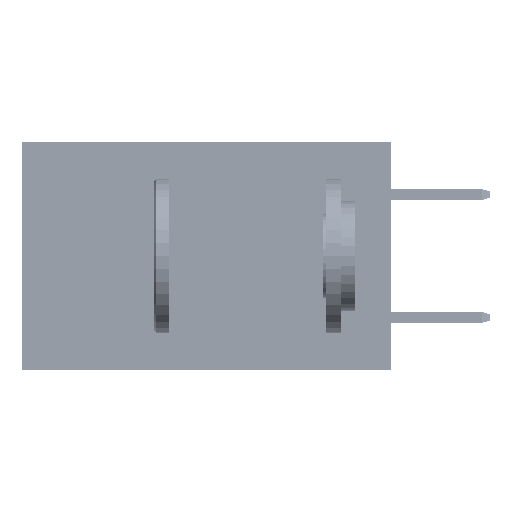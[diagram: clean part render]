
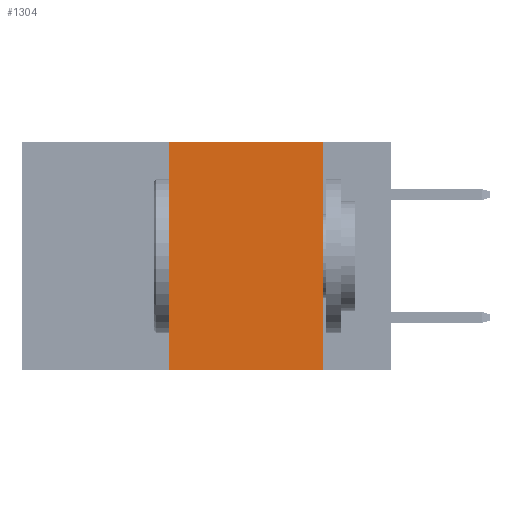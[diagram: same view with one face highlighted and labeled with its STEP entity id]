
A CAD part, left-side view. The second image highlights one B-rep face of the part: STEP entity #1304.
In plain terms, the highlighted planar face has unit normal (-1, 0, 0).
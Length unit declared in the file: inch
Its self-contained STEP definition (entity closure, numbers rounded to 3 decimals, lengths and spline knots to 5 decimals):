
#543 = CARTESIAN_POINT ( 'NONE',  ( 0., 0.6, 0. ) ) ;
#1304 = ADVANCED_FACE ( 'NONE', ( #43577 ), #13617, .F. ) ;
#2218 = DIRECTION ( 'NONE',  ( 0., -1., 0. ) ) ;
#4114 = DIRECTION ( 'NONE',  ( 1., 0., 0. ) ) ;
#5622 = ORIENTED_EDGE ( 'NONE', *, *, #18957, .F. ) ;
#10172 = ORIENTED_EDGE ( 'NONE', *, *, #45277, .F. ) ;
#10402 = LINE ( 'NONE', #49711, #49133 ) ;
#10604 = EDGE_LOOP ( 'NONE', ( #33242, #10172, #5622, #11094 ) ) ;
#11094 = ORIENTED_EDGE ( 'NONE', *, *, #51579, .T. ) ;
#11294 = CARTESIAN_POINT ( 'NONE',  ( 0., 0.11, -0.37 ) ) ;
#11367 = LINE ( 'NONE', #30299, #18952 ) ;
#12908 = CARTESIAN_POINT ( 'NONE',  ( 0., 0.11, 0. ) ) ;
#13617 = PLANE ( 'NONE',  #30441 ) ;
#15164 = CARTESIAN_POINT ( 'NONE',  ( 0., 0.6, 0. ) ) ;
#15316 = LINE ( 'NONE', #20069, #44541 ) ;
#18952 = VECTOR ( 'NONE', #2218, 39.37008 ) ;
#18957 = EDGE_CURVE ( 'NONE', #30375, #23161, #10402, .T. ) ;
#20069 = CARTESIAN_POINT ( 'NONE',  ( 0., 0.11, 0. ) ) ;
#20081 = EDGE_CURVE ( 'NONE', #40708, #21894, #15316, .T. ) ;
#21894 = VERTEX_POINT ( 'NONE', #11294 ) ;
#23161 = VERTEX_POINT ( 'NONE', #42243 ) ;
#27856 = DIRECTION ( 'NONE',  ( 0., 0., -1. ) ) ;
#30299 = CARTESIAN_POINT ( 'NONE',  ( 0., 0.6, -0.37 ) ) ;
#30375 = VERTEX_POINT ( 'NONE', #34197 ) ;
#30441 = AXIS2_PLACEMENT_3D ( 'NONE', #15164, #4114, #50497 ) ;
#33242 = ORIENTED_EDGE ( 'NONE', *, *, #20081, .F. ) ;
#34197 = CARTESIAN_POINT ( 'NONE',  ( 0., 0.36, -0.37 ) ) ;
#37005 = DIRECTION ( 'NONE',  ( 0., -1., 0. ) ) ;
#40708 = VERTEX_POINT ( 'NONE', #12908 ) ;
#40868 = VECTOR ( 'NONE', #37005, 39.37008 ) ;
#41681 = DIRECTION ( 'NONE',  ( 0., 0., 1. ) ) ;
#42243 = CARTESIAN_POINT ( 'NONE',  ( 0., 0.36, 0. ) ) ;
#43577 = FACE_OUTER_BOUND ( 'NONE', #10604, .T. ) ;
#44541 = VECTOR ( 'NONE', #27856, 39.37008 ) ;
#45277 = EDGE_CURVE ( 'NONE', #23161, #40708, #51724, .T. ) ;
#49133 = VECTOR ( 'NONE', #41681, 39.37008 ) ;
#49711 = CARTESIAN_POINT ( 'NONE',  ( 0., 0.36, 0. ) ) ;
#50497 = DIRECTION ( 'NONE',  ( 0., 0., -1. ) ) ;
#51579 = EDGE_CURVE ( 'NONE', #30375, #21894, #11367, .T. ) ;
#51724 = LINE ( 'NONE', #543, #40868 ) ;
